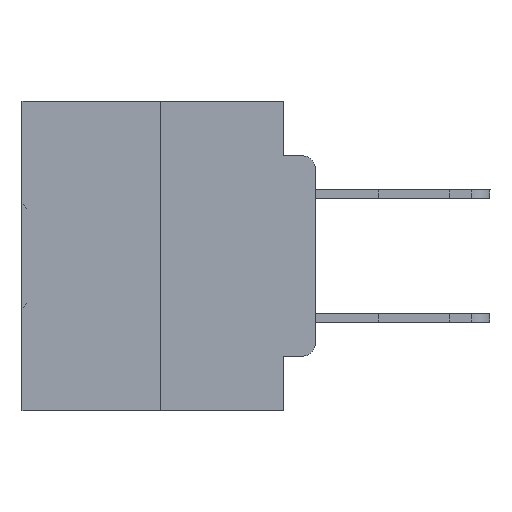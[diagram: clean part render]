
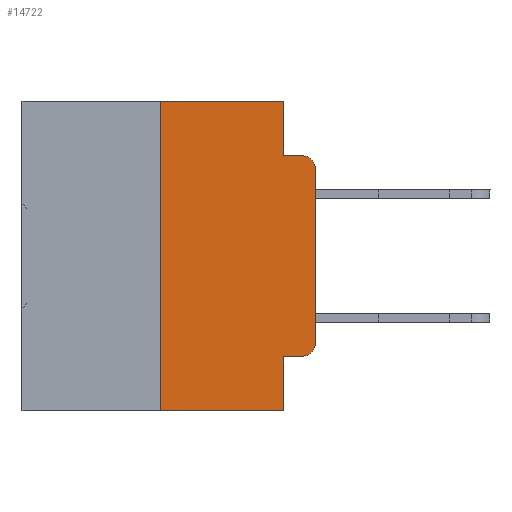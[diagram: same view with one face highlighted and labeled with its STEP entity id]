
A CAD part, left-side view. The second image highlights one B-rep face of the part: STEP entity #14722.
In plain terms, the highlighted planar face has unit normal (-1, 0, 0).
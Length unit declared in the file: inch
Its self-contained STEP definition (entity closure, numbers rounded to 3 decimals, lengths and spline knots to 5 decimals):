
#30 = CARTESIAN_POINT ( 'NONE',  ( 0., 0.051, -0.4115 ) ) ;
#475 = DIRECTION ( 'NONE',  ( 0., 0., -1. ) ) ;
#1976 = EDGE_CURVE ( 'NONE', #6910, #30729, #14505, .T. ) ;
#2188 = CARTESIAN_POINT ( 'NONE',  ( 0., 0.051, -0.5 ) ) ;
#2258 = LINE ( 'NONE', #7739, #23585 ) ;
#2779 = CIRCLE ( 'NONE', #3333, 0.02 ) ;
#2859 = ORIENTED_EDGE ( 'NONE', *, *, #3354, .F. ) ;
#3129 = DIRECTION ( 'NONE',  ( 0., 0., -1. ) ) ;
#3333 = AXIS2_PLACEMENT_3D ( 'NONE', #12541, #14762, #20089 ) ;
#3354 = EDGE_CURVE ( 'NONE', #21762, #24121, #3869, .T. ) ;
#3416 = ORIENTED_EDGE ( 'NONE', *, *, #4256, .T. ) ;
#3570 = DIRECTION ( 'NONE',  ( 0., -1., 0. ) ) ;
#3667 = VECTOR ( 'NONE', #22306, 39.37008 ) ;
#3869 = LINE ( 'NONE', #11597, #24718 ) ;
#4114 = DIRECTION ( 'NONE',  ( 0., 0., -1. ) ) ;
#4256 = EDGE_CURVE ( 'NONE', #21762, #25609, #13076, .T. ) ;
#4394 = CARTESIAN_POINT ( 'NONE',  ( 0., 0.051, -0.0885 ) ) ;
#4493 = VECTOR ( 'NONE', #3570, 39.37008 ) ;
#4521 = EDGE_CURVE ( 'NONE', #25609, #18893, #2779, .T. ) ;
#4745 = EDGE_CURVE ( 'NONE', #14843, #27770, #11477, .T. ) ;
#5695 = PLANE ( 'NONE',  #27308 ) ;
#5703 = EDGE_CURVE ( 'NONE', #13450, #14843, #2258, .T. ) ;
#6146 = ORIENTED_EDGE ( 'NONE', *, *, #5703, .F. ) ;
#6910 = VERTEX_POINT ( 'NONE', #12062 ) ;
#6930 = ORIENTED_EDGE ( 'NONE', *, *, #4521, .T. ) ;
#6981 = CARTESIAN_POINT ( 'NONE',  ( 0., 0., -0.3915 ) ) ;
#7511 = AXIS2_PLACEMENT_3D ( 'NONE', #27119, #14074, #4114 ) ;
#7739 = CARTESIAN_POINT ( 'NONE',  ( 0., 0.25, 0. ) ) ;
#8006 = LINE ( 'NONE', #29492, #8605 ) ;
#8108 = CARTESIAN_POINT ( 'NONE',  ( 0., 0.051, -0.4115 ) ) ;
#8191 = EDGE_CURVE ( 'NONE', #13450, #24121, #14145, .T. ) ;
#8605 = VECTOR ( 'NONE', #475, 39.37008 ) ;
#8760 = CARTESIAN_POINT ( 'NONE',  ( 0., 0.051, 0. ) ) ;
#8898 = CARTESIAN_POINT ( 'NONE',  ( 0., 0.25, -0.5 ) ) ;
#9006 = VERTEX_POINT ( 'NONE', #19374 ) ;
#10503 = DIRECTION ( 'NONE',  ( 0., -1., 0. ) ) ;
#10940 = CARTESIAN_POINT ( 'NONE',  ( 0., 0.02, -0.0885 ) ) ;
#11477 = LINE ( 'NONE', #16456, #4493 ) ;
#11597 = CARTESIAN_POINT ( 'NONE',  ( 0., 0.051, 0. ) ) ;
#11827 = CARTESIAN_POINT ( 'NONE',  ( 0., 0.25, 0. ) ) ;
#12062 = CARTESIAN_POINT ( 'NONE',  ( 0., 0.051, -0.0885 ) ) ;
#12509 = CARTESIAN_POINT ( 'NONE',  ( 0., 0.02, -0.4115 ) ) ;
#12541 = CARTESIAN_POINT ( 'NONE',  ( 0., 0.02, -0.3915 ) ) ;
#12735 = DIRECTION ( 'NONE',  ( 0., 0., 1. ) ) ;
#13076 = LINE ( 'NONE', #30, #20973 ) ;
#13450 = VERTEX_POINT ( 'NONE', #8898 ) ;
#14074 = DIRECTION ( 'NONE',  ( -1., 0., 0. ) ) ;
#14145 = LINE ( 'NONE', #24772, #14481 ) ;
#14481 = VECTOR ( 'NONE', #16906, 39.37008 ) ;
#14505 = LINE ( 'NONE', #4394, #15662 ) ;
#14722 = ADVANCED_FACE ( 'NONE', ( #20961 ), #5695, .F. ) ;
#14762 = DIRECTION ( 'NONE',  ( -1., 0., 0. ) ) ;
#14843 = VERTEX_POINT ( 'NONE', #11827 ) ;
#15577 = ORIENTED_EDGE ( 'NONE', *, *, #30445, .T. ) ;
#15662 = VECTOR ( 'NONE', #29798, 39.37008 ) ;
#16165 = CARTESIAN_POINT ( 'NONE',  ( 0., 0.473, 0. ) ) ;
#16456 = CARTESIAN_POINT ( 'NONE',  ( 0., 0.473, 0. ) ) ;
#16906 = DIRECTION ( 'NONE',  ( 0., -1., 0. ) ) ;
#17341 = ORIENTED_EDGE ( 'NONE', *, *, #4745, .F. ) ;
#17748 = EDGE_LOOP ( 'NONE', ( #18328, #15577, #22578, #19120, #17341, #6146, #24876, #2859, #3416, #6930 ) ) ;
#18328 = ORIENTED_EDGE ( 'NONE', *, *, #30116, .T. ) ;
#18893 = VERTEX_POINT ( 'NONE', #6981 ) ;
#19120 = ORIENTED_EDGE ( 'NONE', *, *, #30698, .F. ) ;
#19374 = CARTESIAN_POINT ( 'NONE',  ( 0., 0., -0.1085 ) ) ;
#20062 = CARTESIAN_POINT ( 'NONE',  ( 0., 0., 0. ) ) ;
#20089 = DIRECTION ( 'NONE',  ( 0., 0., -1. ) ) ;
#20961 = FACE_OUTER_BOUND ( 'NONE', #17748, .T. ) ;
#20973 = VECTOR ( 'NONE', #10503, 39.37008 ) ;
#21762 = VERTEX_POINT ( 'NONE', #8108 ) ;
#22066 = DIRECTION ( 'NONE',  ( 0., 0., -1. ) ) ;
#22306 = DIRECTION ( 'NONE',  ( 0., 0., 1. ) ) ;
#22578 = ORIENTED_EDGE ( 'NONE', *, *, #1976, .F. ) ;
#23585 = VECTOR ( 'NONE', #12735, 39.37008 ) ;
#23935 = CIRCLE ( 'NONE', #7511, 0.02 ) ;
#24121 = VERTEX_POINT ( 'NONE', #2188 ) ;
#24718 = VECTOR ( 'NONE', #22066, 39.37008 ) ;
#24772 = CARTESIAN_POINT ( 'NONE',  ( 0., 0.473, -0.5 ) ) ;
#24876 = ORIENTED_EDGE ( 'NONE', *, *, #8191, .T. ) ;
#25609 = VERTEX_POINT ( 'NONE', #12509 ) ;
#26635 = DIRECTION ( 'NONE',  ( 1., 0., 0. ) ) ;
#27119 = CARTESIAN_POINT ( 'NONE',  ( 0., 0.02, -0.1085 ) ) ;
#27308 = AXIS2_PLACEMENT_3D ( 'NONE', #16165, #26635, #3129 ) ;
#27628 = LINE ( 'NONE', #20062, #3667 ) ;
#27770 = VERTEX_POINT ( 'NONE', #8760 ) ;
#29492 = CARTESIAN_POINT ( 'NONE',  ( 0., 0.051, 0. ) ) ;
#29798 = DIRECTION ( 'NONE',  ( 0., -1., 0. ) ) ;
#30116 = EDGE_CURVE ( 'NONE', #18893, #9006, #27628, .T. ) ;
#30445 = EDGE_CURVE ( 'NONE', #9006, #30729, #23935, .T. ) ;
#30698 = EDGE_CURVE ( 'NONE', #27770, #6910, #8006, .T. ) ;
#30729 = VERTEX_POINT ( 'NONE', #10940 ) ;
